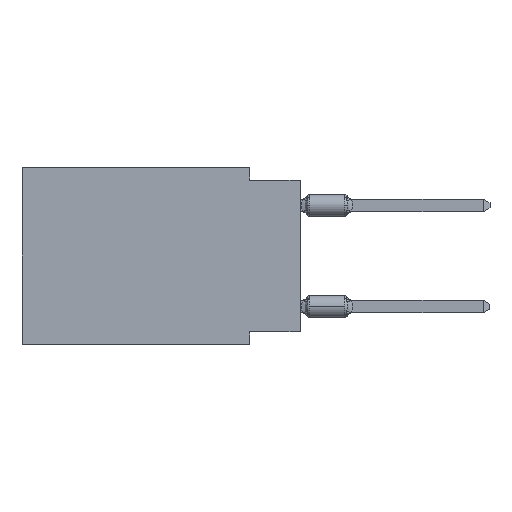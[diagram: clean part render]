
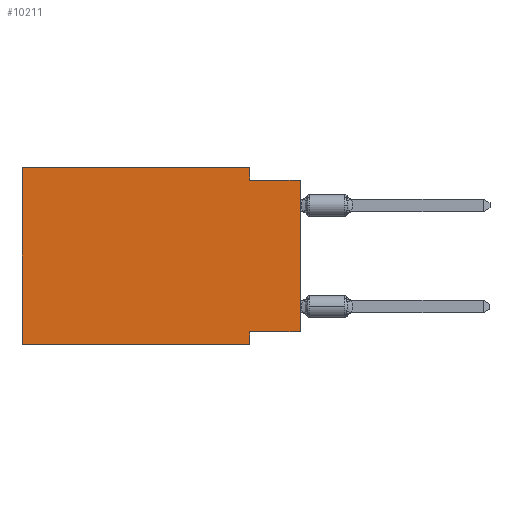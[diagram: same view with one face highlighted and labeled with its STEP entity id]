
A CAD part, left-side view. The second image highlights one B-rep face of the part: STEP entity #10211.
In plain terms, the highlighted planar face has unit normal (-1, 0, 0).
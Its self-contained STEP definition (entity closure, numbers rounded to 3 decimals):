
#48 = EDGE_CURVE ( 'NONE', #8755, #13777, #12709, .T. ) ;
#144 = LINE ( 'NONE', #5991, #12501 ) ;
#237 = ORIENTED_EDGE ( 'NONE', *, *, #9644, .F. ) ;
#244 = EDGE_CURVE ( 'NONE', #12503, #10242, #12448, .T. ) ;
#500 = DIRECTION ( 'NONE',  ( 0., -1., 0. ) ) ;
#747 = ORIENTED_EDGE ( 'NONE', *, *, #11672, .T. ) ;
#866 = LINE ( 'NONE', #10137, #5254 ) ;
#979 = ORIENTED_EDGE ( 'NONE', *, *, #13932, .F. ) ;
#1142 = DIRECTION ( 'NONE',  ( 0., -1., 0. ) ) ;
#1256 = CARTESIAN_POINT ( 'NONE',  ( 0., 0., -8.255 ) ) ;
#1552 = CARTESIAN_POINT ( 'NONE',  ( 0., 13.97, -8.89 ) ) ;
#1983 = CARTESIAN_POINT ( 'NONE',  ( 0., 13.97, -8.89 ) ) ;
#2548 = EDGE_CURVE ( 'NONE', #4762, #10467, #14307, .T. ) ;
#2707 = VERTEX_POINT ( 'NONE', #1983 ) ;
#2814 = DIRECTION ( 'NONE',  ( 1., 0., 0. ) ) ;
#3501 = CARTESIAN_POINT ( 'NONE',  ( 0., 0., -0.635 ) ) ;
#3650 = CARTESIAN_POINT ( 'NONE',  ( 0., 0., -8.255 ) ) ;
#4344 = DIRECTION ( 'NONE',  ( 0., 0., 1. ) ) ;
#4762 = VERTEX_POINT ( 'NONE', #6086 ) ;
#5035 = FACE_OUTER_BOUND ( 'NONE', #10778, .T. ) ;
#5131 = CARTESIAN_POINT ( 'NONE',  ( 0., 13.97, 0. ) ) ;
#5218 = VECTOR ( 'NONE', #500, 1000. ) ;
#5254 = VECTOR ( 'NONE', #4344, 1000. ) ;
#5546 = ORIENTED_EDGE ( 'NONE', *, *, #48, .F. ) ;
#5640 = CARTESIAN_POINT ( 'NONE',  ( 0., 2.54, 0. ) ) ;
#5759 = VECTOR ( 'NONE', #8297, 1000. ) ;
#5867 = LINE ( 'NONE', #3650, #5759 ) ;
#5930 = VERTEX_POINT ( 'NONE', #1256 ) ;
#5991 = CARTESIAN_POINT ( 'NONE',  ( 0., 2.54, 0. ) ) ;
#6086 = CARTESIAN_POINT ( 'NONE',  ( 0., 2.54, -8.255 ) ) ;
#6734 = VECTOR ( 'NONE', #9755, 1000. ) ;
#6756 = ORIENTED_EDGE ( 'NONE', *, *, #2548, .F. ) ;
#6903 = VECTOR ( 'NONE', #8626, 1000. ) ;
#7081 = CARTESIAN_POINT ( 'NONE',  ( 0., 2.54, -8.89 ) ) ;
#7122 = ORIENTED_EDGE ( 'NONE', *, *, #7302, .T. ) ;
#7302 = EDGE_CURVE ( 'NONE', #2707, #10467, #13104, .T. ) ;
#8114 = CARTESIAN_POINT ( 'NONE',  ( 0., 0., -0.635 ) ) ;
#8297 = DIRECTION ( 'NONE',  ( 0., 1., 0. ) ) ;
#8626 = DIRECTION ( 'NONE',  ( 0., 0., 1. ) ) ;
#8755 = VERTEX_POINT ( 'NONE', #14003 ) ;
#8958 = VECTOR ( 'NONE', #1142, 1000. ) ;
#9119 = CARTESIAN_POINT ( 'NONE',  ( 0., 13.97, 0. ) ) ;
#9644 = EDGE_CURVE ( 'NONE', #10242, #8755, #144, .T. ) ;
#9684 = CARTESIAN_POINT ( 'NONE',  ( 0., 13.97, 0. ) ) ;
#9755 = DIRECTION ( 'NONE',  ( 0., 0., -1. ) ) ;
#9923 = DIRECTION ( 'NONE',  ( 0., 0., -1. ) ) ;
#10137 = CARTESIAN_POINT ( 'NONE',  ( 0., 0., 0. ) ) ;
#10211 = ADVANCED_FACE ( 'NONE', ( #5035 ), #13232, .F. ) ;
#10219 = ORIENTED_EDGE ( 'NONE', *, *, #244, .F. ) ;
#10242 = VERTEX_POINT ( 'NONE', #5640 ) ;
#10467 = VERTEX_POINT ( 'NONE', #7081 ) ;
#10778 = EDGE_LOOP ( 'NONE', ( #747, #5546, #237, #10219, #979, #7122, #6756, #14064 ) ) ;
#11672 = EDGE_CURVE ( 'NONE', #5930, #13777, #866, .T. ) ;
#11724 = EDGE_CURVE ( 'NONE', #5930, #4762, #5867, .T. ) ;
#11929 = DIRECTION ( 'NONE',  ( 0., -1., 0. ) ) ;
#12019 = CARTESIAN_POINT ( 'NONE',  ( 0., 2.54, -8.89 ) ) ;
#12048 = LINE ( 'NONE', #5131, #6903 ) ;
#12264 = AXIS2_PLACEMENT_3D ( 'NONE', #9684, #2814, #13619 ) ;
#12448 = LINE ( 'NONE', #9119, #8958 ) ;
#12501 = VECTOR ( 'NONE', #9923, 1000. ) ;
#12503 = VERTEX_POINT ( 'NONE', #12964 ) ;
#12709 = LINE ( 'NONE', #3501, #13328 ) ;
#12964 = CARTESIAN_POINT ( 'NONE',  ( 0., 13.97, 0. ) ) ;
#13104 = LINE ( 'NONE', #1552, #5218 ) ;
#13232 = PLANE ( 'NONE',  #12264 ) ;
#13328 = VECTOR ( 'NONE', #11929, 1000. ) ;
#13619 = DIRECTION ( 'NONE',  ( 0., 0., -1. ) ) ;
#13777 = VERTEX_POINT ( 'NONE', #8114 ) ;
#13932 = EDGE_CURVE ( 'NONE', #2707, #12503, #12048, .T. ) ;
#14003 = CARTESIAN_POINT ( 'NONE',  ( 0., 2.54, -0.635 ) ) ;
#14064 = ORIENTED_EDGE ( 'NONE', *, *, #11724, .F. ) ;
#14307 = LINE ( 'NONE', #12019, #6734 ) ;
